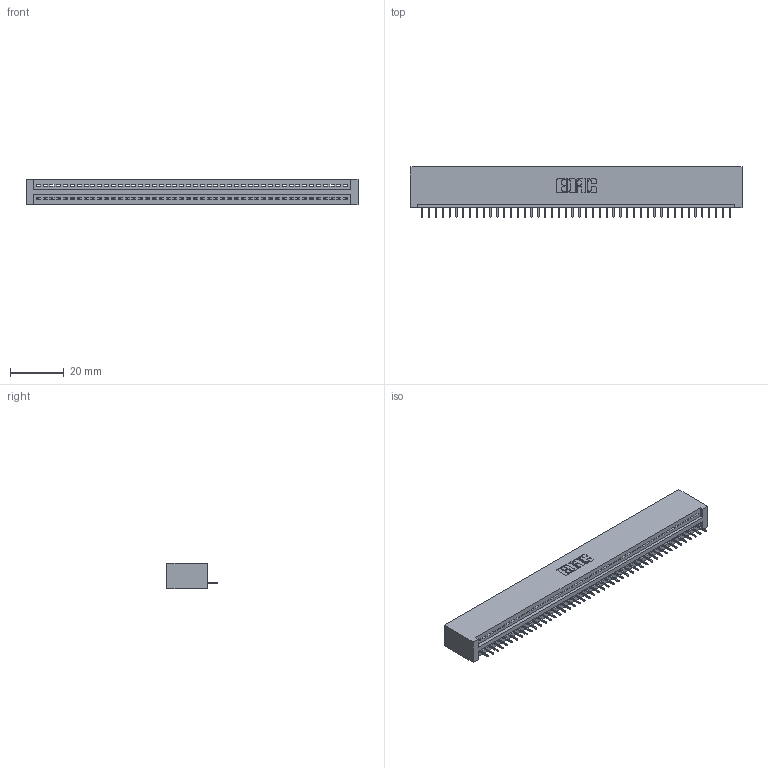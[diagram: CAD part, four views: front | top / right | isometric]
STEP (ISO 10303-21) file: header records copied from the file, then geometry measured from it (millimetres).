
FILE_DESCRIPTION (( 'STEP AP203' ), '1' );
FILE_NAME ('845-046-525-101.STEP', '2020-09-23T07:20:14', ( '' ), ( '' ), 'SwSTEP 2.0', 'SolidWorks 2020', '' );
FILE_SCHEMA (( 'CONFIG_CONTROL_DESIGN' ));
Length unit declared in the file: inch
Products named in the file (3): 845-046-525-101; 845 Part_No Mounting Lugs; 345-292-001_345-293-125
Assembly tree (47 placements, depth 2):
  845-046-525-101
    845 Part_No Mounting Lugs
    345-292-001_345-293-125  x46
Bounding box: 123.44 x 18.72 x 9.4 mm (x, y, z)
Volume: 12154.1 mm3; surface area: 15770 mm2
Topology: 47 solids, 47 shells, 2970 faces, 8597 edges, 5546 vertices
Faces by surface type: plane 2192, cylinder 778
Entity records: 33879 total; most frequent: CARTESIAN_POINT 5874, ORIENTED_EDGE 5854, DIRECTION 5119, EDGE_CURVE 2927, VECTOR 2623, LINE 2623, VERTEX_POINT 1946, AXIS2_PLACEMENT_3D 1248
